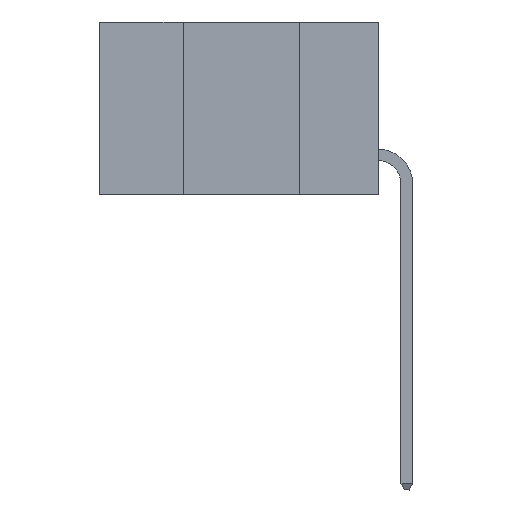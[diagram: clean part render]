
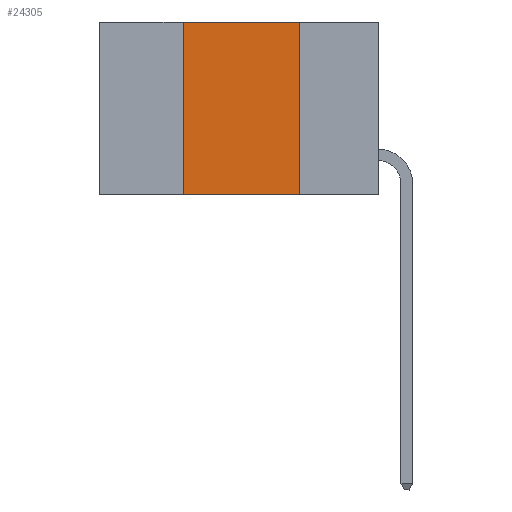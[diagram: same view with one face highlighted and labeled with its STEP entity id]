
A CAD part, left-side view. The second image highlights one B-rep face of the part: STEP entity #24305.
In plain terms, the highlighted planar face has unit normal (-1, 0, 0).
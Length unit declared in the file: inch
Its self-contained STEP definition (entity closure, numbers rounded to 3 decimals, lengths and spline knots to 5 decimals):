
#353 = LINE ( 'NONE', #20077, #11037 ) ;
#431 = VECTOR ( 'NONE', #28271, 39.37008 ) ;
#1040 = CARTESIAN_POINT ( 'NONE',  ( 0., 0.42, 0. ) ) ;
#1522 = CARTESIAN_POINT ( 'NONE',  ( 0., 0.6, 0. ) ) ;
#1906 = EDGE_LOOP ( 'NONE', ( #5524, #18454, #1949, #17927 ) ) ;
#1949 = ORIENTED_EDGE ( 'NONE', *, *, #29362, .F. ) ;
#2157 = DIRECTION ( 'NONE',  ( 0., 0., -1. ) ) ;
#2865 = VERTEX_POINT ( 'NONE', #16901 ) ;
#3064 = EDGE_CURVE ( 'NONE', #13347, #11090, #8103, .T. ) ;
#3175 = EDGE_CURVE ( 'NONE', #2865, #15932, #27764, .T. ) ;
#3329 = CARTESIAN_POINT ( 'NONE',  ( 0., 0.42, 0. ) ) ;
#4734 = DIRECTION ( 'NONE',  ( 1., 0., 0. ) ) ;
#5524 = ORIENTED_EDGE ( 'NONE', *, *, #10167, .F. ) ;
#6128 = DIRECTION ( 'NONE',  ( 0., -1., 0. ) ) ;
#6635 = DIRECTION ( 'NONE',  ( 0., -1., 0. ) ) ;
#7736 = VECTOR ( 'NONE', #6635, 39.37008 ) ;
#8103 = LINE ( 'NONE', #1522, #29548 ) ;
#10167 = EDGE_CURVE ( 'NONE', #11090, #15932, #353, .T. ) ;
#11037 = VECTOR ( 'NONE', #26600, 39.37008 ) ;
#11090 = VERTEX_POINT ( 'NONE', #11427 ) ;
#11427 = CARTESIAN_POINT ( 'NONE',  ( 0., 0.17, 0. ) ) ;
#13273 = LINE ( 'NONE', #1040, #431 ) ;
#13347 = VERTEX_POINT ( 'NONE', #3329 ) ;
#13702 = CARTESIAN_POINT ( 'NONE',  ( 0., 0.6, 0. ) ) ;
#15932 = VERTEX_POINT ( 'NONE', #28760 ) ;
#16901 = CARTESIAN_POINT ( 'NONE',  ( 0., 0.42, -0.37 ) ) ;
#17927 = ORIENTED_EDGE ( 'NONE', *, *, #3175, .T. ) ;
#18454 = ORIENTED_EDGE ( 'NONE', *, *, #3064, .F. ) ;
#19502 = FACE_OUTER_BOUND ( 'NONE', #1906, .T. ) ;
#20077 = CARTESIAN_POINT ( 'NONE',  ( 0., 0.17, 0. ) ) ;
#20094 = CARTESIAN_POINT ( 'NONE',  ( 0., 0.6, -0.37 ) ) ;
#24305 = ADVANCED_FACE ( 'NONE', ( #19502 ), #25115, .F. ) ;
#25115 = PLANE ( 'NONE',  #25670 ) ;
#25670 = AXIS2_PLACEMENT_3D ( 'NONE', #13702, #4734, #2157 ) ;
#26600 = DIRECTION ( 'NONE',  ( 0., 0., -1. ) ) ;
#27764 = LINE ( 'NONE', #20094, #7736 ) ;
#28271 = DIRECTION ( 'NONE',  ( 0., 0., 1. ) ) ;
#28760 = CARTESIAN_POINT ( 'NONE',  ( 0., 0.17, -0.37 ) ) ;
#29362 = EDGE_CURVE ( 'NONE', #2865, #13347, #13273, .T. ) ;
#29548 = VECTOR ( 'NONE', #6128, 39.37008 ) ;
